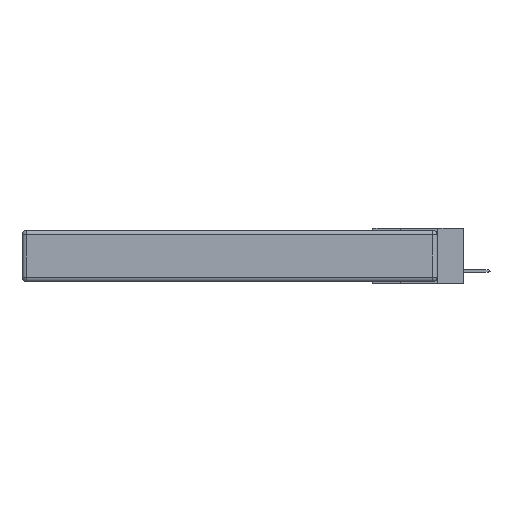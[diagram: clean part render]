
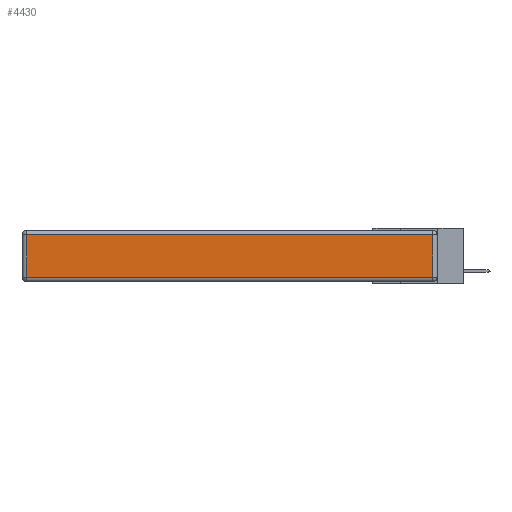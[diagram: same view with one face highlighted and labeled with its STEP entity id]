
A CAD part, left-side view. The second image highlights one B-rep face of the part: STEP entity #4430.
In plain terms, the highlighted planar face has unit normal (-1, 0, 0).
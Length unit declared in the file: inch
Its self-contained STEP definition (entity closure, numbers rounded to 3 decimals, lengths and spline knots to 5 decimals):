
#228 = DIRECTION ( 'NONE',  ( 0., 0., 1. ) ) ;
#882 = CARTESIAN_POINT ( 'NONE',  ( 0., 0., -0.343 ) ) ;
#915 = EDGE_CURVE ( 'NONE', #11615, #13258, #3785, .T. ) ;
#1291 = VECTOR ( 'NONE', #13626, 39.37008 ) ;
#1377 = CARTESIAN_POINT ( 'NONE',  ( 0., 0.03, -0.313 ) ) ;
#2743 = PLANE ( 'NONE',  #21690 ) ;
#3182 = VECTOR ( 'NONE', #228, 39.37008 ) ;
#3559 = CARTESIAN_POINT ( 'NONE',  ( 0., 0.03, -0.03 ) ) ;
#3785 = LINE ( 'NONE', #18249, #3182 ) ;
#3995 = ORIENTED_EDGE ( 'NONE', *, *, #7658, .T. ) ;
#4430 = ADVANCED_FACE ( 'NONE', ( #21834 ), #2743, .T. ) ;
#5719 = DIRECTION ( 'NONE',  ( 0., 1., 0. ) ) ;
#5939 = ORIENTED_EDGE ( 'NONE', *, *, #915, .T. ) ;
#6197 = LINE ( 'NONE', #23027, #12115 ) ;
#7658 = EDGE_CURVE ( 'NONE', #18539, #11615, #24786, .T. ) ;
#8204 = ORIENTED_EDGE ( 'NONE', *, *, #9924, .T. ) ;
#9924 = EDGE_CURVE ( 'NONE', #13258, #14643, #18793, .T. ) ;
#11145 = EDGE_LOOP ( 'NONE', ( #3995, #5939, #8204, #20190 ) ) ;
#11174 = DIRECTION ( 'NONE',  ( 0., 0., -1. ) ) ;
#11615 = VERTEX_POINT ( 'NONE', #1377 ) ;
#12115 = VECTOR ( 'NONE', #11174, 39.37008 ) ;
#13155 = EDGE_CURVE ( 'NONE', #14643, #18539, #6197, .T. ) ;
#13258 = VERTEX_POINT ( 'NONE', #3559 ) ;
#13545 = CARTESIAN_POINT ( 'NONE',  ( 0., 0., -0.313 ) ) ;
#13626 = DIRECTION ( 'NONE',  ( 0., -1., 0. ) ) ;
#14643 = VERTEX_POINT ( 'NONE', #23655 ) ;
#15660 = VECTOR ( 'NONE', #5719, 39.37008 ) ;
#17420 = CARTESIAN_POINT ( 'NONE',  ( 0., 2.72, -0.313 ) ) ;
#18249 = CARTESIAN_POINT ( 'NONE',  ( 0., 0.03, -0.343 ) ) ;
#18539 = VERTEX_POINT ( 'NONE', #17420 ) ;
#18553 = DIRECTION ( 'NONE',  ( 0., 0., 1. ) ) ;
#18727 = DIRECTION ( 'NONE',  ( -1., 0., 0. ) ) ;
#18793 = LINE ( 'NONE', #19376, #15660 ) ;
#19376 = CARTESIAN_POINT ( 'NONE',  ( 0., 2.75, -0.03 ) ) ;
#20190 = ORIENTED_EDGE ( 'NONE', *, *, #13155, .T. ) ;
#21690 = AXIS2_PLACEMENT_3D ( 'NONE', #882, #18727, #18553 ) ;
#21834 = FACE_OUTER_BOUND ( 'NONE', #11145, .T. ) ;
#23027 = CARTESIAN_POINT ( 'NONE',  ( 0., 2.72, -0.343 ) ) ;
#23655 = CARTESIAN_POINT ( 'NONE',  ( 0., 2.72, -0.03 ) ) ;
#24786 = LINE ( 'NONE', #13545, #1291 ) ;
